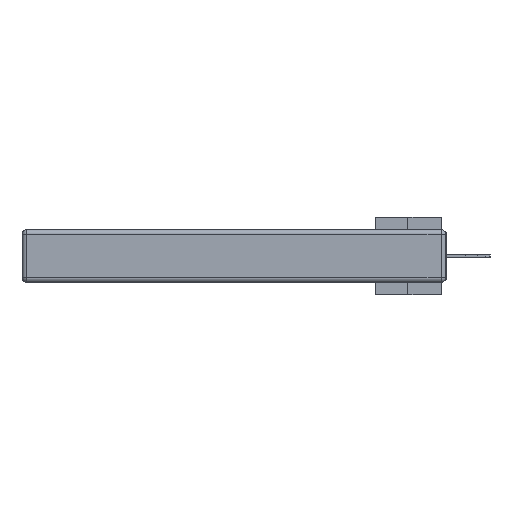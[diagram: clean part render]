
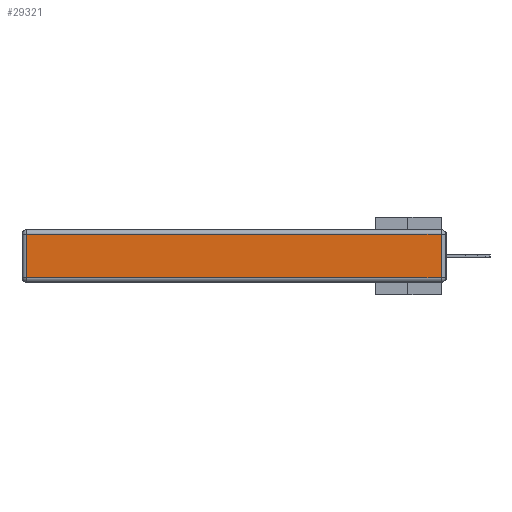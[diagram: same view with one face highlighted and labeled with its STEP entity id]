
A CAD part, left-side view. The second image highlights one B-rep face of the part: STEP entity #29321.
In plain terms, the highlighted planar face has unit normal (-1, 0, 0).
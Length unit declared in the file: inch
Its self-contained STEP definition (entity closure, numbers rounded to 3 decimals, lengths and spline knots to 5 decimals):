
#2081 = LINE ( 'NONE', #33571, #23121 ) ;
#2380 = EDGE_CURVE ( 'NONE', #11363, #25245, #2081, .T. ) ;
#3932 = VERTEX_POINT ( 'NONE', #18287 ) ;
#4297 = DIRECTION ( 'NONE',  ( 0., -1., 0. ) ) ;
#5888 = CARTESIAN_POINT ( 'NONE',  ( 0., 0., -0.343 ) ) ;
#8602 = EDGE_CURVE ( 'NONE', #3932, #33879, #29784, .T. ) ;
#9420 = CARTESIAN_POINT ( 'NONE',  ( 0., 0., -0.313 ) ) ;
#10192 = DIRECTION ( 'NONE',  ( 0., 1., 0. ) ) ;
#11363 = VERTEX_POINT ( 'NONE', #13717 ) ;
#12830 = DIRECTION ( 'NONE',  ( 0., 0., 1. ) ) ;
#13717 = CARTESIAN_POINT ( 'NONE',  ( 0., 0.03, -0.03 ) ) ;
#14768 = PLANE ( 'NONE',  #26478 ) ;
#15125 = VECTOR ( 'NONE', #12830, 39.37008 ) ;
#15672 = VECTOR ( 'NONE', #28931, 39.37008 ) ;
#16127 = CARTESIAN_POINT ( 'NONE',  ( 0., 0.03, -0.313 ) ) ;
#16651 = ORIENTED_EDGE ( 'NONE', *, *, #8602, .T. ) ;
#17429 = LINE ( 'NONE', #37052, #15672 ) ;
#17622 = ORIENTED_EDGE ( 'NONE', *, *, #2380, .T. ) ;
#18287 = CARTESIAN_POINT ( 'NONE',  ( 0., 2.72, -0.313 ) ) ;
#21615 = EDGE_LOOP ( 'NONE', ( #16651, #30957, #17622, #34602 ) ) ;
#23068 = FACE_OUTER_BOUND ( 'NONE', #21615, .T. ) ;
#23121 = VECTOR ( 'NONE', #10192, 39.37008 ) ;
#23257 = CARTESIAN_POINT ( 'NONE',  ( 0., 2.72, -0.03 ) ) ;
#23615 = DIRECTION ( 'NONE',  ( -1., 0., 0. ) ) ;
#23631 = EDGE_CURVE ( 'NONE', #25245, #3932, #17429, .T. ) ;
#24130 = LINE ( 'NONE', #35633, #15125 ) ;
#24814 = VECTOR ( 'NONE', #4297, 39.37008 ) ;
#25245 = VERTEX_POINT ( 'NONE', #23257 ) ;
#26478 = AXIS2_PLACEMENT_3D ( 'NONE', #5888, #23615, #37186 ) ;
#28931 = DIRECTION ( 'NONE',  ( 0., 0., -1. ) ) ;
#29321 = ADVANCED_FACE ( 'NONE', ( #23068 ), #14768, .T. ) ;
#29784 = LINE ( 'NONE', #9420, #24814 ) ;
#30526 = EDGE_CURVE ( 'NONE', #33879, #11363, #24130, .T. ) ;
#30957 = ORIENTED_EDGE ( 'NONE', *, *, #30526, .T. ) ;
#33571 = CARTESIAN_POINT ( 'NONE',  ( 0., 2.75, -0.03 ) ) ;
#33879 = VERTEX_POINT ( 'NONE', #16127 ) ;
#34602 = ORIENTED_EDGE ( 'NONE', *, *, #23631, .T. ) ;
#35633 = CARTESIAN_POINT ( 'NONE',  ( 0., 0.03, -0.343 ) ) ;
#37052 = CARTESIAN_POINT ( 'NONE',  ( 0., 2.72, -0.343 ) ) ;
#37186 = DIRECTION ( 'NONE',  ( 0., 0., 1. ) ) ;
